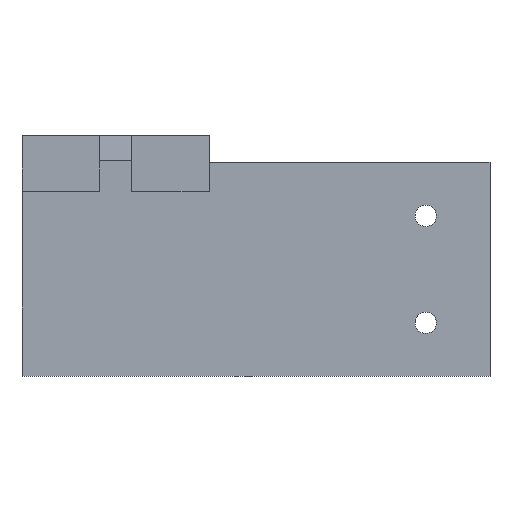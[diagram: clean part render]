
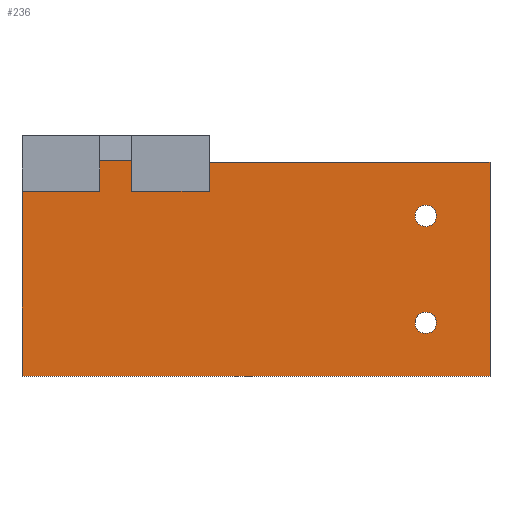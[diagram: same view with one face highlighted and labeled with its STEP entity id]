
A CAD part, top view. The second image highlights one B-rep face of the part: STEP entity #236.
In plain terms, the highlighted planar face has unit normal (0, 0, 1).
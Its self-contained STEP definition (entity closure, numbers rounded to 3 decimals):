
#4 = LINE ( 'NONE', #737, #336 ) ;
#15 = ORIENTED_EDGE ( 'NONE', *, *, #756, .T. ) ;
#26 = VERTEX_POINT ( 'NONE', #1137 ) ;
#28 = DIRECTION ( 'NONE',  ( -1., 0., 0. ) ) ;
#45 = EDGE_CURVE ( 'NONE', #26, #821, #651, .T. ) ;
#46 = EDGE_LOOP ( 'NONE', ( #523, #858 ) ) ;
#59 = CARTESIAN_POINT ( 'NONE',  ( -14., 10., 12. ) ) ;
#61 = CARTESIAN_POINT ( 'NONE',  ( -73., 20.337, 12. ) ) ;
#65 = CARTESIAN_POINT ( 'NONE',  ( -10., 10., 12. ) ) ;
#70 = CIRCLE ( 'NONE', #1073, 2. ) ;
#92 = VECTOR ( 'NONE', #234, 1000. ) ;
#103 = DIRECTION ( 'NONE',  ( 0., 0., 1. ) ) ;
#138 = CARTESIAN_POINT ( 'NONE',  ( -73., 14.574, 12. ) ) ;
#146 = DIRECTION ( 'NONE',  ( 0., 0., 1. ) ) ;
#154 = DIRECTION ( 'NONE',  ( 0., 0., -1. ) ) ;
#172 = EDGE_CURVE ( 'NONE', #1087, #1093, #1092, .T. ) ;
#173 = EDGE_CURVE ( 'NONE', #1093, #1087, #70, .T. ) ;
#175 = ORIENTED_EDGE ( 'NONE', *, *, #635, .F. ) ;
#187 = CARTESIAN_POINT ( 'NONE',  ( -73., 14.574, 12. ) ) ;
#189 = CARTESIAN_POINT ( 'NONE',  ( -87.5, 14.574, 12. ) ) ;
#194 = ORIENTED_EDGE ( 'NONE', *, *, #977, .T. ) ;
#197 = VERTEX_POINT ( 'NONE', #779 ) ;
#198 = AXIS2_PLACEMENT_3D ( 'NONE', #926, #256, #270 ) ;
#215 = DIRECTION ( 'NONE',  ( 1., 0., 0. ) ) ;
#225 = ORIENTED_EDGE ( 'NONE', *, *, #777, .F. ) ;
#229 = CARTESIAN_POINT ( 'NONE',  ( -10., -10., 12. ) ) ;
#231 = DIRECTION ( 'NONE',  ( 0., 0., 1. ) ) ;
#234 = DIRECTION ( 'NONE',  ( 0., -1., 0. ) ) ;
#236 = ADVANCED_FACE ( 'NONE', ( #530, #1010, #984 ), #265, .F. ) ;
#239 = DIRECTION ( 'NONE',  ( 0., -1., 0. ) ) ;
#247 = CARTESIAN_POINT ( 'NONE',  ( -14., -10., 12. ) ) ;
#248 = DIRECTION ( 'NONE',  ( 1., 0., 0. ) ) ;
#251 = DIRECTION ( 'NONE',  ( -1., 0., 0. ) ) ;
#256 = DIRECTION ( 'NONE',  ( 0., 0., 1. ) ) ;
#261 = VECTOR ( 'NONE', #950, 1000. ) ;
#264 = VERTEX_POINT ( 'NONE', #624 ) ;
#265 = PLANE ( 'NONE',  #903 ) ;
#270 = DIRECTION ( 'NONE',  ( 1., 0., 0. ) ) ;
#293 = DIRECTION ( 'NONE',  ( 0., -1., 0. ) ) ;
#305 = VECTOR ( 'NONE', #1081, 1000. ) ;
#325 = CARTESIAN_POINT ( 'NONE',  ( -67., 20., 12. ) ) ;
#336 = VECTOR ( 'NONE', #461, 1000. ) ;
#341 = LINE ( 'NONE', #711, #305 ) ;
#347 = LINE ( 'NONE', #325, #92 ) ;
#354 = DIRECTION ( 'NONE',  ( -1., 0., 0. ) ) ;
#358 = EDGE_CURVE ( 'NONE', #387, #688, #534, .T. ) ;
#381 = EDGE_CURVE ( 'NONE', #853, #1082, #388, .T. ) ;
#387 = VERTEX_POINT ( 'NONE', #1034 ) ;
#388 = LINE ( 'NONE', #1103, #865 ) ;
#410 = EDGE_LOOP ( 'NONE', ( #1056, #1112, #1134, #15, #684, #194, #550, #580, #1069, #785 ) ) ;
#445 = CARTESIAN_POINT ( 'NONE',  ( -67., 20.337, 12. ) ) ;
#457 = EDGE_CURVE ( 'NONE', #688, #26, #4, .T. ) ;
#461 = DIRECTION ( 'NONE',  ( -1., 0., 0. ) ) ;
#470 = AXIS2_PLACEMENT_3D ( 'NONE', #692, #146, #215 ) ;
#471 = DIRECTION ( 'NONE',  ( 1., 0., 0. ) ) ;
#484 = LINE ( 'NONE', #187, #1013 ) ;
#485 = VERTEX_POINT ( 'NONE', #189 ) ;
#507 = EDGE_CURVE ( 'NONE', #892, #853, #731, .T. ) ;
#523 = ORIENTED_EDGE ( 'NONE', *, *, #173, .F. ) ;
#530 = FACE_OUTER_BOUND ( 'NONE', #410, .T. ) ;
#534 = LINE ( 'NONE', #920, #1186 ) ;
#550 = ORIENTED_EDGE ( 'NONE', *, *, #358, .T. ) ;
#572 = VECTOR ( 'NONE', #248, 1000. ) ;
#576 = CARTESIAN_POINT ( 'NONE',  ( -12., 10., 12. ) ) ;
#580 = ORIENTED_EDGE ( 'NONE', *, *, #457, .T. ) ;
#621 = CARTESIAN_POINT ( 'NONE',  ( 0., -20., 12. ) ) ;
#624 = CARTESIAN_POINT ( 'NONE',  ( -87.5, -20., 12. ) ) ;
#635 = EDGE_CURVE ( 'NONE', #966, #945, #994, .T. ) ;
#644 = CARTESIAN_POINT ( 'NONE',  ( -52.5, 20., 12. ) ) ;
#651 = LINE ( 'NONE', #644, #261 ) ;
#684 = ORIENTED_EDGE ( 'NONE', *, *, #1151, .T. ) ;
#688 = VERTEX_POINT ( 'NONE', #946 ) ;
#692 = CARTESIAN_POINT ( 'NONE',  ( -12., -10., 12. ) ) ;
#706 = CARTESIAN_POINT ( 'NONE',  ( 0., 0., 12. ) ) ;
#711 = CARTESIAN_POINT ( 'NONE',  ( -67., 14.574, 12. ) ) ;
#714 = AXIS2_PLACEMENT_3D ( 'NONE', #576, #103, #471 ) ;
#731 = LINE ( 'NONE', #811, #1071 ) ;
#737 = CARTESIAN_POINT ( 'NONE',  ( 0., 20., 12. ) ) ;
#756 = EDGE_CURVE ( 'NONE', #1082, #485, #484, .T. ) ;
#768 = VECTOR ( 'NONE', #239, 1000. ) ;
#777 = EDGE_CURVE ( 'NONE', #945, #966, #888, .T. ) ;
#779 = CARTESIAN_POINT ( 'NONE',  ( -67., 14.574, 12. ) ) ;
#785 = ORIENTED_EDGE ( 'NONE', *, *, #1183, .F. ) ;
#809 = LINE ( 'NONE', #1075, #768 ) ;
#811 = CARTESIAN_POINT ( 'NONE',  ( 0., 20.337, 12. ) ) ;
#821 = VERTEX_POINT ( 'NONE', #981 ) ;
#840 = EDGE_LOOP ( 'NONE', ( #175, #225 ) ) ;
#853 = VERTEX_POINT ( 'NONE', #61 ) ;
#858 = ORIENTED_EDGE ( 'NONE', *, *, #172, .F. ) ;
#865 = VECTOR ( 'NONE', #293, 1000. ) ;
#888 = CIRCLE ( 'NONE', #714, 2. ) ;
#889 = DIRECTION ( 'NONE',  ( 1., 0., 0. ) ) ;
#892 = VERTEX_POINT ( 'NONE', #445 ) ;
#903 = AXIS2_PLACEMENT_3D ( 'NONE', #706, #154, #251 ) ;
#920 = CARTESIAN_POINT ( 'NONE',  ( 0., 20., 12. ) ) ;
#926 = CARTESIAN_POINT ( 'NONE',  ( -12., 10., 12. ) ) ;
#945 = VERTEX_POINT ( 'NONE', #65 ) ;
#946 = CARTESIAN_POINT ( 'NONE',  ( 0., 20., 12. ) ) ;
#950 = DIRECTION ( 'NONE',  ( 0., -1., 0. ) ) ;
#966 = VERTEX_POINT ( 'NONE', #59 ) ;
#977 = EDGE_CURVE ( 'NONE', #264, #387, #1178, .T. ) ;
#981 = CARTESIAN_POINT ( 'NONE',  ( -52.5, 14.574, 12. ) ) ;
#984 = FACE_BOUND ( 'NONE', #46, .T. ) ;
#994 = CIRCLE ( 'NONE', #198, 2. ) ;
#1010 = FACE_BOUND ( 'NONE', #840, .T. ) ;
#1013 = VECTOR ( 'NONE', #28, 1000. ) ;
#1034 = CARTESIAN_POINT ( 'NONE',  ( 0., -20., 12. ) ) ;
#1056 = ORIENTED_EDGE ( 'NONE', *, *, #1143, .F. ) ;
#1063 = CARTESIAN_POINT ( 'NONE',  ( -12., -10., 12. ) ) ;
#1069 = ORIENTED_EDGE ( 'NONE', *, *, #45, .T. ) ;
#1071 = VECTOR ( 'NONE', #354, 1000. ) ;
#1073 = AXIS2_PLACEMENT_3D ( 'NONE', #1063, #231, #889 ) ;
#1075 = CARTESIAN_POINT ( 'NONE',  ( -87.5, 20., 12. ) ) ;
#1081 = DIRECTION ( 'NONE',  ( 1., 0., 0. ) ) ;
#1082 = VERTEX_POINT ( 'NONE', #138 ) ;
#1087 = VERTEX_POINT ( 'NONE', #229 ) ;
#1092 = CIRCLE ( 'NONE', #470, 2. ) ;
#1093 = VERTEX_POINT ( 'NONE', #247 ) ;
#1103 = CARTESIAN_POINT ( 'NONE',  ( -73., 14.574, 12. ) ) ;
#1112 = ORIENTED_EDGE ( 'NONE', *, *, #507, .T. ) ;
#1134 = ORIENTED_EDGE ( 'NONE', *, *, #381, .T. ) ;
#1137 = CARTESIAN_POINT ( 'NONE',  ( -52.5, 20., 12. ) ) ;
#1143 = EDGE_CURVE ( 'NONE', #892, #197, #347, .T. ) ;
#1151 = EDGE_CURVE ( 'NONE', #485, #264, #809, .T. ) ;
#1168 = DIRECTION ( 'NONE',  ( 0., 1., 0. ) ) ;
#1178 = LINE ( 'NONE', #621, #572 ) ;
#1183 = EDGE_CURVE ( 'NONE', #197, #821, #341, .T. ) ;
#1186 = VECTOR ( 'NONE', #1168, 1000. ) ;
